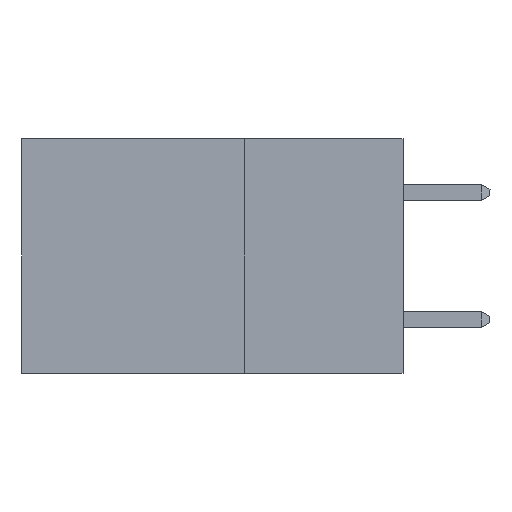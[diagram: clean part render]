
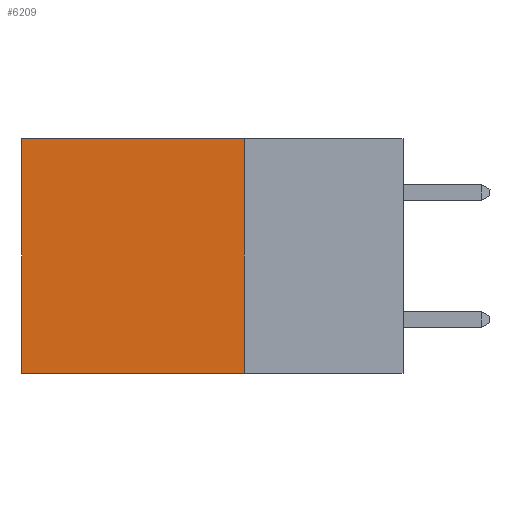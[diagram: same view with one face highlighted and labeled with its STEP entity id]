
A CAD part, left-side view. The second image highlights one B-rep face of the part: STEP entity #6209.
In plain terms, the highlighted planar face has unit normal (-1, 0, 0).
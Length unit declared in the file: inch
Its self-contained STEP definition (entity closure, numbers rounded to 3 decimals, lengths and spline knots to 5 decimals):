
#241 = EDGE_LOOP ( 'NONE', ( #14518, #7352, #5555, #5454 ) ) ;
#980 = DIRECTION ( 'NONE',  ( 0., 0., -1. ) ) ;
#1114 = VECTOR ( 'NONE', #980, 39.37008 ) ;
#1637 = CARTESIAN_POINT ( 'NONE',  ( 0.2875, 0.6, -0.37 ) ) ;
#1736 = CARTESIAN_POINT ( 'NONE',  ( 0.2875, 0.25, 0. ) ) ;
#3668 = CARTESIAN_POINT ( 'NONE',  ( 0.2875, 0.25, 0. ) ) ;
#3793 = CARTESIAN_POINT ( 'NONE',  ( 0.2875, 0.25, 0. ) ) ;
#3803 = EDGE_CURVE ( 'NONE', #5876, #14674, #8234, .T. ) ;
#4195 = CARTESIAN_POINT ( 'NONE',  ( 0.2875, 0.6, 0. ) ) ;
#4233 = FACE_OUTER_BOUND ( 'NONE', #241, .T. ) ;
#4686 = DIRECTION ( 'NONE',  ( 0., 1., 0. ) ) ;
#5114 = DIRECTION ( 'NONE',  ( 0., 0., -1. ) ) ;
#5307 = EDGE_CURVE ( 'NONE', #5876, #8854, #7158, .T. ) ;
#5454 = ORIENTED_EDGE ( 'NONE', *, *, #5307, .T. ) ;
#5555 = ORIENTED_EDGE ( 'NONE', *, *, #3803, .F. ) ;
#5782 = VECTOR ( 'NONE', #14919, 39.37008 ) ;
#5876 = VERTEX_POINT ( 'NONE', #1736 ) ;
#6209 = ADVANCED_FACE ( 'NONE', ( #4233 ), #13023, .F. ) ;
#6721 = AXIS2_PLACEMENT_3D ( 'NONE', #3793, #13134, #5114 ) ;
#6958 = CARTESIAN_POINT ( 'NONE',  ( 0.2875, 0.25, -0.37 ) ) ;
#7158 = LINE ( 'NONE', #12711, #15777 ) ;
#7352 = ORIENTED_EDGE ( 'NONE', *, *, #10402, .F. ) ;
#8234 = LINE ( 'NONE', #3668, #1114 ) ;
#8854 = VERTEX_POINT ( 'NONE', #9726 ) ;
#9074 = LINE ( 'NONE', #4195, #12684 ) ;
#9726 = CARTESIAN_POINT ( 'NONE',  ( 0.2875, 0.6, 0. ) ) ;
#10402 = EDGE_CURVE ( 'NONE', #14674, #14528, #12908, .T. ) ;
#11085 = EDGE_CURVE ( 'NONE', #8854, #14528, #9074, .T. ) ;
#12684 = VECTOR ( 'NONE', #14843, 39.37008 ) ;
#12711 = CARTESIAN_POINT ( 'NONE',  ( 0.2875, 0.25, 0. ) ) ;
#12908 = LINE ( 'NONE', #6958, #5782 ) ;
#13023 = PLANE ( 'NONE',  #6721 ) ;
#13134 = DIRECTION ( 'NONE',  ( 1., 0., 0. ) ) ;
#14518 = ORIENTED_EDGE ( 'NONE', *, *, #11085, .T. ) ;
#14528 = VERTEX_POINT ( 'NONE', #1637 ) ;
#14674 = VERTEX_POINT ( 'NONE', #15219 ) ;
#14843 = DIRECTION ( 'NONE',  ( 0., 0., -1. ) ) ;
#14919 = DIRECTION ( 'NONE',  ( 0., 1., 0. ) ) ;
#15219 = CARTESIAN_POINT ( 'NONE',  ( 0.2875, 0.25, -0.37 ) ) ;
#15777 = VECTOR ( 'NONE', #4686, 39.37008 ) ;
